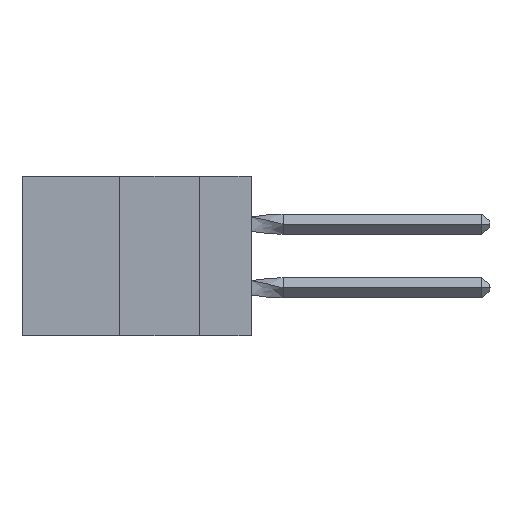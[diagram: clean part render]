
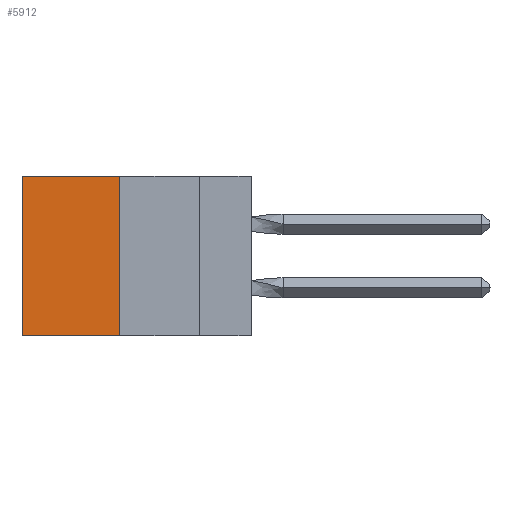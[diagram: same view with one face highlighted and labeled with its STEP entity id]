
A CAD part, left-side view. The second image highlights one B-rep face of the part: STEP entity #5912.
In plain terms, the highlighted planar face has unit normal (-1, 0, 0).
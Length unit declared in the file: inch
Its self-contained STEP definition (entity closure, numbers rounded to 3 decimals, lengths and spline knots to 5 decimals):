
#956 = ORIENTED_EDGE ( 'NONE', *, *, #11500, .T. ) ;
#1921 = EDGE_CURVE ( 'NONE', #2888, #29459, #25800, .T. ) ;
#2152 = CARTESIAN_POINT ( 'NONE',  ( 0.305, 0.413, -0.5 ) ) ;
#2318 = CARTESIAN_POINT ( 'NONE',  ( 0.305, 0.72, -0.5 ) ) ;
#2657 = LINE ( 'NONE', #8892, #35866 ) ;
#2888 = VERTEX_POINT ( 'NONE', #36241 ) ;
#5912 = ADVANCED_FACE ( 'NONE', ( #22091 ), #11450, .F. ) ;
#6002 = AXIS2_PLACEMENT_3D ( 'NONE', #11026, #33013, #17447 ) ;
#8892 = CARTESIAN_POINT ( 'NONE',  ( 0.305, 0.413, 0. ) ) ;
#11026 = CARTESIAN_POINT ( 'NONE',  ( 0.305, 0.413, -0.5 ) ) ;
#11450 = PLANE ( 'NONE',  #6002 ) ;
#11500 = EDGE_CURVE ( 'NONE', #16133, #11763, #2657, .T. ) ;
#11763 = VERTEX_POINT ( 'NONE', #23617 ) ;
#16133 = VERTEX_POINT ( 'NONE', #30240 ) ;
#16290 = LINE ( 'NONE', #31311, #20247 ) ;
#17314 = EDGE_LOOP ( 'NONE', ( #25449, #39829, #32476, #956 ) ) ;
#17447 = DIRECTION ( 'NONE',  ( 0., 0., -1. ) ) ;
#18075 = DIRECTION ( 'NONE',  ( 0., 1., 0. ) ) ;
#19008 = CARTESIAN_POINT ( 'NONE',  ( 0.305, 0.72, -0.5 ) ) ;
#19861 = EDGE_CURVE ( 'NONE', #16133, #2888, #16290, .T. ) ;
#20247 = VECTOR ( 'NONE', #40964, 39.37008 ) ;
#22091 = FACE_OUTER_BOUND ( 'NONE', #17314, .T. ) ;
#22805 = EDGE_CURVE ( 'NONE', #11763, #29459, #25868, .T. ) ;
#23617 = CARTESIAN_POINT ( 'NONE',  ( 0.305, 0.72, 0. ) ) ;
#25449 = ORIENTED_EDGE ( 'NONE', *, *, #22805, .T. ) ;
#25800 = LINE ( 'NONE', #2152, #28250 ) ;
#25868 = LINE ( 'NONE', #2318, #40167 ) ;
#27641 = DIRECTION ( 'NONE',  ( 0., 1., 0. ) ) ;
#28250 = VECTOR ( 'NONE', #27641, 39.37008 ) ;
#29459 = VERTEX_POINT ( 'NONE', #19008 ) ;
#30240 = CARTESIAN_POINT ( 'NONE',  ( 0.305, 0.413, 0. ) ) ;
#31311 = CARTESIAN_POINT ( 'NONE',  ( 0.305, 0.413, -0.5 ) ) ;
#32476 = ORIENTED_EDGE ( 'NONE', *, *, #19861, .F. ) ;
#33013 = DIRECTION ( 'NONE',  ( 1., 0., 0. ) ) ;
#35866 = VECTOR ( 'NONE', #18075, 39.37008 ) ;
#36241 = CARTESIAN_POINT ( 'NONE',  ( 0.305, 0.413, -0.5 ) ) ;
#37163 = DIRECTION ( 'NONE',  ( 0., 0., -1. ) ) ;
#39829 = ORIENTED_EDGE ( 'NONE', *, *, #1921, .F. ) ;
#40167 = VECTOR ( 'NONE', #37163, 39.37008 ) ;
#40964 = DIRECTION ( 'NONE',  ( 0., 0., -1. ) ) ;
